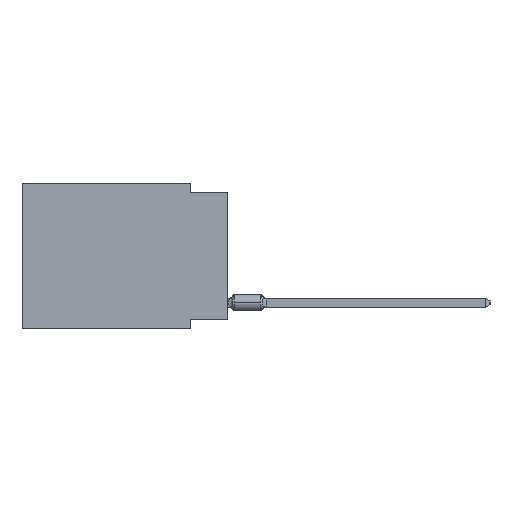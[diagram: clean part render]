
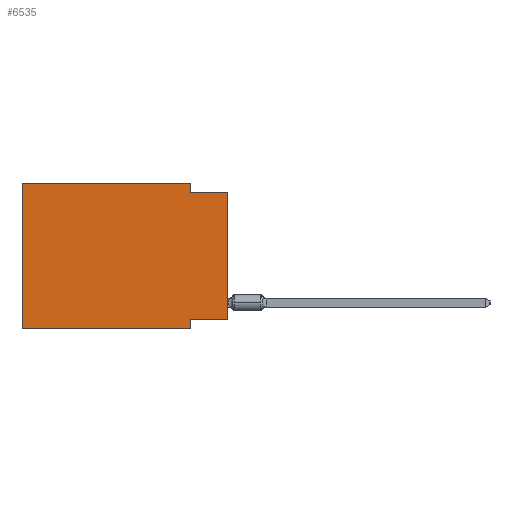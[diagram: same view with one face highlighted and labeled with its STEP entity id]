
A CAD part, left-side view. The second image highlights one B-rep face of the part: STEP entity #6535.
In plain terms, the highlighted planar face has unit normal (-1, 0, 0).
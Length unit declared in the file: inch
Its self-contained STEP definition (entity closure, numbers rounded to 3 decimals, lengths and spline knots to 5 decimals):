
#19 = ORIENTED_EDGE ( 'NONE', *, *, #13541, .F. ) ;
#1991 = EDGE_CURVE ( 'NONE', #9687, #41402, #9796, .T. ) ;
#3242 = DIRECTION ( 'NONE',  ( 0., 0., -1. ) ) ;
#3812 = ORIENTED_EDGE ( 'NONE', *, *, #24325, .T. ) ;
#4080 = LINE ( 'NONE', #33549, #49223 ) ;
#6535 = ADVANCED_FACE ( 'NONE', ( #8382 ), #47308, .F. ) ;
#6828 = ORIENTED_EDGE ( 'NONE', *, *, #20385, .F. ) ;
#8007 = DIRECTION ( 'NONE',  ( 0., 0., -1. ) ) ;
#8172 = VECTOR ( 'NONE', #8007, 39.37008 ) ;
#8382 = FACE_OUTER_BOUND ( 'NONE', #48120, .T. ) ;
#9687 = VERTEX_POINT ( 'NONE', #42821 ) ;
#9796 = LINE ( 'NONE', #15188, #50148 ) ;
#10156 = DIRECTION ( 'NONE',  ( 0., 0., 1. ) ) ;
#10199 = AXIS2_PLACEMENT_3D ( 'NONE', #52188, #13250, #3242 ) ;
#10440 = VECTOR ( 'NONE', #10156, 39.37008 ) ;
#12284 = CARTESIAN_POINT ( 'NONE',  ( 0., 0.1, -0.39 ) ) ;
#12613 = VERTEX_POINT ( 'NONE', #26932 ) ;
#12897 = VERTEX_POINT ( 'NONE', #55774 ) ;
#12970 = VECTOR ( 'NONE', #26271, 39.37008 ) ;
#13243 = ORIENTED_EDGE ( 'NONE', *, *, #33748, .T. ) ;
#13250 = DIRECTION ( 'NONE',  ( 1., 0., 0. ) ) ;
#13541 = EDGE_CURVE ( 'NONE', #16158, #12613, #14173, .T. ) ;
#13614 = EDGE_CURVE ( 'NONE', #41402, #18973, #54235, .T. ) ;
#14173 = LINE ( 'NONE', #22769, #10440 ) ;
#15188 = CARTESIAN_POINT ( 'NONE',  ( 0., 0.1, 0. ) ) ;
#16158 = VERTEX_POINT ( 'NONE', #24285 ) ;
#18973 = VERTEX_POINT ( 'NONE', #42819 ) ;
#20233 = VECTOR ( 'NONE', #51206, 39.37008 ) ;
#20385 = EDGE_CURVE ( 'NONE', #55825, #12897, #22019, .T. ) ;
#20899 = ORIENTED_EDGE ( 'NONE', *, *, #21151, .F. ) ;
#21151 = EDGE_CURVE ( 'NONE', #41885, #55825, #53991, .T. ) ;
#22019 = LINE ( 'NONE', #12284, #8172 ) ;
#22769 = CARTESIAN_POINT ( 'NONE',  ( 0., 0.55, 0. ) ) ;
#23050 = DIRECTION ( 'NONE',  ( 0., -1., 0. ) ) ;
#24285 = CARTESIAN_POINT ( 'NONE',  ( 0., 0.55, -0.39 ) ) ;
#24325 = EDGE_CURVE ( 'NONE', #16158, #12897, #42927, .T. ) ;
#26271 = DIRECTION ( 'NONE',  ( 0., -1., 0. ) ) ;
#26875 = ORIENTED_EDGE ( 'NONE', *, *, #1991, .F. ) ;
#26932 = CARTESIAN_POINT ( 'NONE',  ( 0., 0.55, 0. ) ) ;
#27131 = CARTESIAN_POINT ( 'NONE',  ( 0., 0., -0.365 ) ) ;
#28285 = CARTESIAN_POINT ( 'NONE',  ( 0., 0.1, -0.365 ) ) ;
#28773 = CARTESIAN_POINT ( 'NONE',  ( 0., 0., -0.365 ) ) ;
#29921 = ORIENTED_EDGE ( 'NONE', *, *, #13614, .F. ) ;
#30248 = ORIENTED_EDGE ( 'NONE', *, *, #39528, .F. ) ;
#31557 = DIRECTION ( 'NONE',  ( 0., 0., -1. ) ) ;
#32913 = VECTOR ( 'NONE', #46219, 39.37008 ) ;
#33549 = CARTESIAN_POINT ( 'NONE',  ( 0., 0., 0. ) ) ;
#33748 = EDGE_CURVE ( 'NONE', #41885, #18973, #4080, .T. ) ;
#33754 = CARTESIAN_POINT ( 'NONE',  ( 0., 0.55, -0.39 ) ) ;
#39528 = EDGE_CURVE ( 'NONE', #12613, #9687, #49127, .T. ) ;
#41402 = VERTEX_POINT ( 'NONE', #47577 ) ;
#41885 = VERTEX_POINT ( 'NONE', #27131 ) ;
#42413 = VECTOR ( 'NONE', #23050, 39.37008 ) ;
#42819 = CARTESIAN_POINT ( 'NONE',  ( 0., 0., -0.025 ) ) ;
#42821 = CARTESIAN_POINT ( 'NONE',  ( 0., 0.1, 0. ) ) ;
#42927 = LINE ( 'NONE', #33754, #20233 ) ;
#46219 = DIRECTION ( 'NONE',  ( 0., 1., 0. ) ) ;
#46701 = DIRECTION ( 'NONE',  ( 0., 0., 1. ) ) ;
#47308 = PLANE ( 'NONE',  #10199 ) ;
#47577 = CARTESIAN_POINT ( 'NONE',  ( 0., 0.1, -0.025 ) ) ;
#48120 = EDGE_LOOP ( 'NONE', ( #13243, #29921, #26875, #30248, #19, #3812, #6828, #20899 ) ) ;
#49127 = LINE ( 'NONE', #53144, #12970 ) ;
#49223 = VECTOR ( 'NONE', #46701, 39.37008 ) ;
#49374 = CARTESIAN_POINT ( 'NONE',  ( 0., 0., -0.025 ) ) ;
#50148 = VECTOR ( 'NONE', #31557, 39.37008 ) ;
#51206 = DIRECTION ( 'NONE',  ( 0., -1., 0. ) ) ;
#52188 = CARTESIAN_POINT ( 'NONE',  ( 0., 0.55, 0. ) ) ;
#53144 = CARTESIAN_POINT ( 'NONE',  ( 0., 0.55, 0. ) ) ;
#53991 = LINE ( 'NONE', #28773, #32913 ) ;
#54235 = LINE ( 'NONE', #49374, #42413 ) ;
#55774 = CARTESIAN_POINT ( 'NONE',  ( 0., 0.1, -0.39 ) ) ;
#55825 = VERTEX_POINT ( 'NONE', #28285 ) ;
